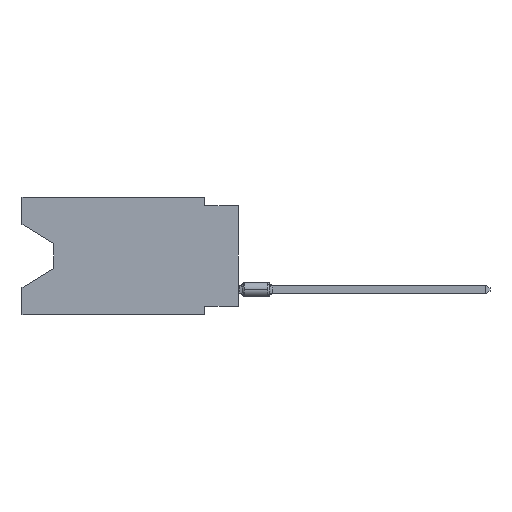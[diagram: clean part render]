
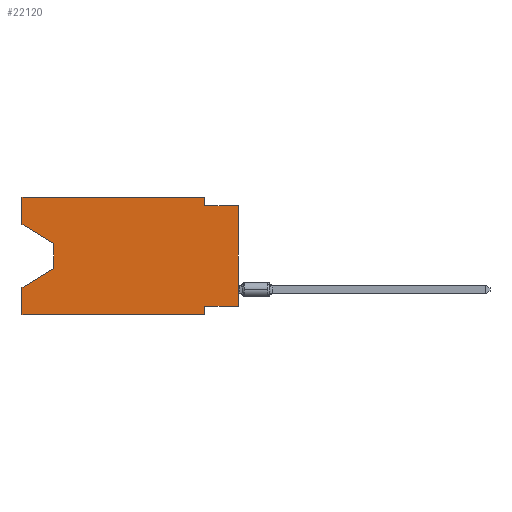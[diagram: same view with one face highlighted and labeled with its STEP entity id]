
A CAD part, left-side view. The second image highlights one B-rep face of the part: STEP entity #22120.
In plain terms, the highlighted planar face has unit normal (-1, 0, 0).
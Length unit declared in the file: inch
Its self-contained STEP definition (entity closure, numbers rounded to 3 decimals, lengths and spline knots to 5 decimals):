
#88 = DIRECTION ( 'NONE',  ( 0., 0., -1. ) ) ;
#128 = DIRECTION ( 'NONE',  ( 0., -1., 0. ) ) ;
#852 = CARTESIAN_POINT ( 'NONE',  ( 0., 0.1, -0.35 ) ) ;
#1060 = VERTEX_POINT ( 'NONE', #11328 ) ;
#1269 = CARTESIAN_POINT ( 'NONE',  ( 0., 0.55, -0.138 ) ) ;
#2021 = VECTOR ( 'NONE', #15139, 39.37008 ) ;
#2256 = DIRECTION ( 'NONE',  ( 0., 0.855, -0.519 ) ) ;
#3381 = DIRECTION ( 'NONE',  ( 0., 0., 1. ) ) ;
#3811 = VECTOR ( 'NONE', #2256, 39.37008 ) ;
#3978 = DIRECTION ( 'NONE',  ( 0., 0., -1. ) ) ;
#4455 = VECTOR ( 'NONE', #23073, 39.37008 ) ;
#4522 = LINE ( 'NONE', #11985, #27918 ) ;
#5548 = LINE ( 'NONE', #8149, #26322 ) ;
#6059 = VECTOR ( 'NONE', #88, 39.37008 ) ;
#6857 = EDGE_CURVE ( 'NONE', #27188, #7457, #17310, .T. ) ;
#7457 = VERTEX_POINT ( 'NONE', #27099 ) ;
#7602 = LINE ( 'NONE', #17175, #31411 ) ;
#7803 = ORIENTED_EDGE ( 'NONE', *, *, #13587, .F. ) ;
#8149 = CARTESIAN_POINT ( 'NONE',  ( 0., 0.645, 0. ) ) ;
#8292 = EDGE_CURVE ( 'NONE', #28584, #16894, #5548, .T. ) ;
#8386 = VERTEX_POINT ( 'NONE', #21272 ) ;
#9012 = VECTOR ( 'NONE', #10002, 39.37008 ) ;
#10002 = DIRECTION ( 'NONE',  ( 0., 0., -1. ) ) ;
#10078 = EDGE_CURVE ( 'NONE', #8386, #18887, #24465, .T. ) ;
#10140 = CARTESIAN_POINT ( 'NONE',  ( 0., 0.55, -0.138 ) ) ;
#10434 = CARTESIAN_POINT ( 'NONE',  ( 0., 0.1, -0.025 ) ) ;
#11328 = CARTESIAN_POINT ( 'NONE',  ( 0., 0., -0.325 ) ) ;
#11346 = CARTESIAN_POINT ( 'NONE',  ( 0., 0., 0. ) ) ;
#11394 = CARTESIAN_POINT ( 'NONE',  ( 0., 0.645, -0.26975 ) ) ;
#11920 = PLANE ( 'NONE',  #26015 ) ;
#11985 = CARTESIAN_POINT ( 'NONE',  ( 0., 0.645, 0. ) ) ;
#12259 = CARTESIAN_POINT ( 'NONE',  ( 0., 0.1, 0. ) ) ;
#12328 = ORIENTED_EDGE ( 'NONE', *, *, #23921, .F. ) ;
#12961 = EDGE_CURVE ( 'NONE', #17098, #7457, #23070, .T. ) ;
#13098 = VECTOR ( 'NONE', #3381, 39.37008 ) ;
#13105 = DIRECTION ( 'NONE',  ( 0., 0., 1. ) ) ;
#13587 = EDGE_CURVE ( 'NONE', #29097, #28584, #4522, .T. ) ;
#13705 = EDGE_CURVE ( 'NONE', #1060, #17098, #24140, .T. ) ;
#13954 = ORIENTED_EDGE ( 'NONE', *, *, #22771, .T. ) ;
#14133 = CARTESIAN_POINT ( 'NONE',  ( 0., 0.645, 0. ) ) ;
#15139 = DIRECTION ( 'NONE',  ( 0., 0., -1. ) ) ;
#16310 = CARTESIAN_POINT ( 'NONE',  ( 0., 0.645, 0. ) ) ;
#16894 = VERTEX_POINT ( 'NONE', #29722 ) ;
#17079 = VECTOR ( 'NONE', #13105, 39.37008 ) ;
#17098 = VERTEX_POINT ( 'NONE', #18359 ) ;
#17175 = CARTESIAN_POINT ( 'NONE',  ( 0., 0.645, -0.08025 ) ) ;
#17310 = LINE ( 'NONE', #24769, #25981 ) ;
#17493 = DIRECTION ( 'NONE',  ( 0., -0.855, -0.519 ) ) ;
#17651 = CARTESIAN_POINT ( 'NONE',  ( 0., 0.55, -0.212 ) ) ;
#18238 = EDGE_CURVE ( 'NONE', #24402, #22288, #25185, .T. ) ;
#18310 = LINE ( 'NONE', #11346, #13098 ) ;
#18359 = CARTESIAN_POINT ( 'NONE',  ( 0., 0.1, -0.325 ) ) ;
#18813 = ORIENTED_EDGE ( 'NONE', *, *, #6857, .T. ) ;
#18887 = VERTEX_POINT ( 'NONE', #11394 ) ;
#18936 = LINE ( 'NONE', #12259, #9012 ) ;
#19043 = EDGE_CURVE ( 'NONE', #29097, #23711, #7602, .T. ) ;
#19125 = ORIENTED_EDGE ( 'NONE', *, *, #8292, .F. ) ;
#19365 = FACE_OUTER_BOUND ( 'NONE', #24308, .T. ) ;
#20177 = CARTESIAN_POINT ( 'NONE',  ( 0., 0., -0.025 ) ) ;
#20378 = ORIENTED_EDGE ( 'NONE', *, *, #10078, .T. ) ;
#20589 = ORIENTED_EDGE ( 'NONE', *, *, #21084, .T. ) ;
#20923 = CARTESIAN_POINT ( 'NONE',  ( 0., 0.645, -0.35 ) ) ;
#21084 = EDGE_CURVE ( 'NONE', #23711, #8386, #29748, .T. ) ;
#21272 = CARTESIAN_POINT ( 'NONE',  ( 0., 0.55, -0.212 ) ) ;
#21714 = CARTESIAN_POINT ( 'NONE',  ( 0., 0., -0.325 ) ) ;
#21798 = DIRECTION ( 'NONE',  ( 1., 0., 0. ) ) ;
#22120 = ADVANCED_FACE ( 'NONE', ( #19365 ), #11920, .F. ) ;
#22288 = VERTEX_POINT ( 'NONE', #29414 ) ;
#22771 = EDGE_CURVE ( 'NONE', #1060, #22288, #18310, .T. ) ;
#23070 = LINE ( 'NONE', #852, #2021 ) ;
#23073 = DIRECTION ( 'NONE',  ( 0., -1., 0. ) ) ;
#23711 = VERTEX_POINT ( 'NONE', #1269 ) ;
#23921 = EDGE_CURVE ( 'NONE', #16894, #24402, #18936, .T. ) ;
#24140 = LINE ( 'NONE', #21714, #28953 ) ;
#24308 = EDGE_LOOP ( 'NONE', ( #25302, #20589, #20378, #28365, #18813, #29574, #28850, #13954, #24760, #12328, #19125, #7803 ) ) ;
#24402 = VERTEX_POINT ( 'NONE', #10434 ) ;
#24465 = LINE ( 'NONE', #17651, #3811 ) ;
#24760 = ORIENTED_EDGE ( 'NONE', *, *, #18238, .F. ) ;
#24769 = CARTESIAN_POINT ( 'NONE',  ( 0., 0.645, -0.35 ) ) ;
#25185 = LINE ( 'NONE', #20177, #4455 ) ;
#25302 = ORIENTED_EDGE ( 'NONE', *, *, #19043, .T. ) ;
#25981 = VECTOR ( 'NONE', #128, 39.37008 ) ;
#26015 = AXIS2_PLACEMENT_3D ( 'NONE', #16310, #21798, #3978 ) ;
#26322 = VECTOR ( 'NONE', #27440, 39.37008 ) ;
#27099 = CARTESIAN_POINT ( 'NONE',  ( 0., 0.1, -0.35 ) ) ;
#27188 = VERTEX_POINT ( 'NONE', #20923 ) ;
#27440 = DIRECTION ( 'NONE',  ( 0., -1., 0. ) ) ;
#27517 = EDGE_CURVE ( 'NONE', #27188, #18887, #30129, .T. ) ;
#27532 = CARTESIAN_POINT ( 'NONE',  ( 0., 0.645, 0. ) ) ;
#27918 = VECTOR ( 'NONE', #31304, 39.37008 ) ;
#28365 = ORIENTED_EDGE ( 'NONE', *, *, #27517, .F. ) ;
#28584 = VERTEX_POINT ( 'NONE', #14133 ) ;
#28850 = ORIENTED_EDGE ( 'NONE', *, *, #13705, .F. ) ;
#28953 = VECTOR ( 'NONE', #31611, 39.37008 ) ;
#29097 = VERTEX_POINT ( 'NONE', #30498 ) ;
#29414 = CARTESIAN_POINT ( 'NONE',  ( 0., 0., -0.025 ) ) ;
#29574 = ORIENTED_EDGE ( 'NONE', *, *, #12961, .F. ) ;
#29722 = CARTESIAN_POINT ( 'NONE',  ( 0., 0.1, 0. ) ) ;
#29748 = LINE ( 'NONE', #10140, #6059 ) ;
#30129 = LINE ( 'NONE', #27532, #17079 ) ;
#30498 = CARTESIAN_POINT ( 'NONE',  ( 0., 0.645, -0.08025 ) ) ;
#31304 = DIRECTION ( 'NONE',  ( 0., 0., 1. ) ) ;
#31411 = VECTOR ( 'NONE', #17493, 39.37008 ) ;
#31611 = DIRECTION ( 'NONE',  ( 0., 1., 0. ) ) ;
